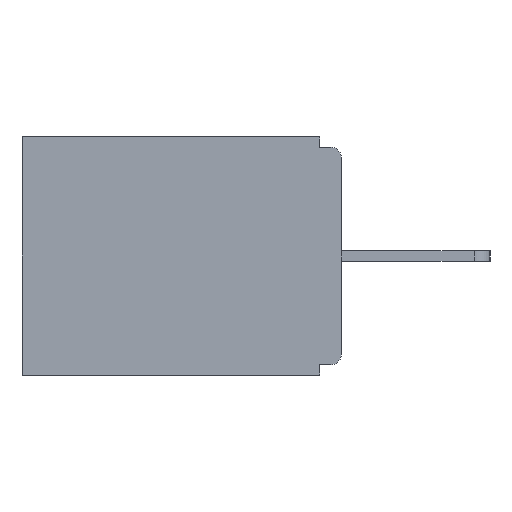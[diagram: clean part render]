
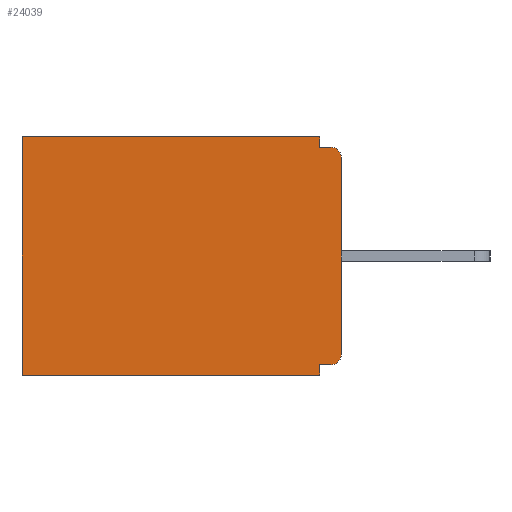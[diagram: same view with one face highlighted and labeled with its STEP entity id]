
A CAD part, left-side view. The second image highlights one B-rep face of the part: STEP entity #24039.
In plain terms, the highlighted planar face has unit normal (-1, 0, 0).
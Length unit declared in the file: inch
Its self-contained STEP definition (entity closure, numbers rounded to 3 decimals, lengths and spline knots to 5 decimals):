
#53 = LINE ( 'NONE', #6033, #4845 ) ;
#126 = VECTOR ( 'NONE', #24595, 39.37008 ) ;
#134 = EDGE_LOOP ( 'NONE', ( #587, #21879, #17811, #18312, #21061, #21093, #11610, #23595, #15843, #8886 ) ) ;
#587 = ORIENTED_EDGE ( 'NONE', *, *, #18206, .T. ) ;
#593 = CARTESIAN_POINT ( 'NONE',  ( 0.298, 0.015, -0.328 ) ) ;
#1632 = EDGE_CURVE ( 'NONE', #15498, #21610, #16433, .T. ) ;
#1956 = VECTOR ( 'NONE', #16701, 39.37008 ) ;
#2041 = VERTEX_POINT ( 'NONE', #22790 ) ;
#2462 = DIRECTION ( 'NONE',  ( 0., 0., -1. ) ) ;
#2502 = VERTEX_POINT ( 'NONE', #20215 ) ;
#3595 = EDGE_CURVE ( 'NONE', #24499, #2502, #21696, .T. ) ;
#3769 = FACE_OUTER_BOUND ( 'NONE', #134, .T. ) ;
#4038 = PLANE ( 'NONE',  #14611 ) ;
#4407 = EDGE_CURVE ( 'NONE', #12067, #2502, #9379, .T. ) ;
#4606 = CARTESIAN_POINT ( 'NONE',  ( 0.298, 0.031, 0. ) ) ;
#4625 = EDGE_CURVE ( 'NONE', #16371, #12067, #24307, .T. ) ;
#4845 = VECTOR ( 'NONE', #13504, 39.37008 ) ;
#4949 = VECTOR ( 'NONE', #23212, 39.37008 ) ;
#6033 = CARTESIAN_POINT ( 'NONE',  ( 0.298, 0.031, -0.343 ) ) ;
#6102 = DIRECTION ( 'NONE',  ( 0., 0., -1. ) ) ;
#6248 = EDGE_CURVE ( 'NONE', #18153, #21610, #20789, .T. ) ;
#6457 = CARTESIAN_POINT ( 'NONE',  ( 0.298, 0., 0. ) ) ;
#6572 = DIRECTION ( 'NONE',  ( 0., 1., 0. ) ) ;
#6909 = EDGE_CURVE ( 'NONE', #2041, #24272, #15732, .T. ) ;
#7142 = CARTESIAN_POINT ( 'NONE',  ( 0.298, 0., -0.328 ) ) ;
#7146 = CARTESIAN_POINT ( 'NONE',  ( 0.298, 0., -0.03 ) ) ;
#7517 = AXIS2_PLACEMENT_3D ( 'NONE', #8905, #22947, #10972 ) ;
#7763 = EDGE_CURVE ( 'NONE', #16371, #2041, #53, .T. ) ;
#7942 = CARTESIAN_POINT ( 'NONE',  ( 0.298, 0.015, -0.313 ) ) ;
#8074 = VECTOR ( 'NONE', #2462, 39.37008 ) ;
#8426 = VERTEX_POINT ( 'NONE', #22854 ) ;
#8474 = DIRECTION ( 'NONE',  ( 0., 0., -1. ) ) ;
#8886 = ORIENTED_EDGE ( 'NONE', *, *, #1632, .F. ) ;
#8905 = CARTESIAN_POINT ( 'NONE',  ( 0.298, 0.015, -0.03 ) ) ;
#9199 = EDGE_CURVE ( 'NONE', #8426, #24499, #18119, .T. ) ;
#9379 = LINE ( 'NONE', #12613, #8074 ) ;
#10373 = VECTOR ( 'NONE', #16014, 39.37008 ) ;
#10446 = CARTESIAN_POINT ( 'NONE',  ( 0.298, 0.031, -0.343 ) ) ;
#10972 = DIRECTION ( 'NONE',  ( 0., 0., -1. ) ) ;
#11020 = CARTESIAN_POINT ( 'NONE',  ( 0.298, 0.015, -0.015 ) ) ;
#11089 = VECTOR ( 'NONE', #8474, 39.37008 ) ;
#11223 = CARTESIAN_POINT ( 'NONE',  ( 0.298, 0., 0. ) ) ;
#11610 = ORIENTED_EDGE ( 'NONE', *, *, #9199, .F. ) ;
#12067 = VERTEX_POINT ( 'NONE', #25063 ) ;
#12613 = CARTESIAN_POINT ( 'NONE',  ( 0.298, 0.46, 0. ) ) ;
#13504 = DIRECTION ( 'NONE',  ( 0., 0., -1. ) ) ;
#14611 = AXIS2_PLACEMENT_3D ( 'NONE', #25976, #18225, #6102 ) ;
#15498 = VERTEX_POINT ( 'NONE', #7146 ) ;
#15732 = LINE ( 'NONE', #17384, #10373 ) ;
#15843 = ORIENTED_EDGE ( 'NONE', *, *, #6248, .T. ) ;
#15930 = AXIS2_PLACEMENT_3D ( 'NONE', #7942, #21995, #25230 ) ;
#16014 = DIRECTION ( 'NONE',  ( 0., -1., 0. ) ) ;
#16371 = VERTEX_POINT ( 'NONE', #4606 ) ;
#16433 = LINE ( 'NONE', #11223, #11089 ) ;
#16701 = DIRECTION ( 'NONE',  ( 0., 0., -1. ) ) ;
#17384 = CARTESIAN_POINT ( 'NONE',  ( 0.298, 0., -0.015 ) ) ;
#17642 = EDGE_CURVE ( 'NONE', #18153, #8426, #21115, .T. ) ;
#17770 = CARTESIAN_POINT ( 'NONE',  ( 0.298, 0.031, -0.343 ) ) ;
#17811 = ORIENTED_EDGE ( 'NONE', *, *, #7763, .F. ) ;
#18119 = LINE ( 'NONE', #10446, #1956 ) ;
#18153 = VERTEX_POINT ( 'NONE', #593 ) ;
#18206 = EDGE_CURVE ( 'NONE', #15498, #24272, #24113, .T. ) ;
#18225 = DIRECTION ( 'NONE',  ( 1., 0., 0. ) ) ;
#18312 = ORIENTED_EDGE ( 'NONE', *, *, #4625, .T. ) ;
#19141 = VECTOR ( 'NONE', #6572, 39.37008 ) ;
#20215 = CARTESIAN_POINT ( 'NONE',  ( 0.298, 0.46, -0.343 ) ) ;
#20695 = CARTESIAN_POINT ( 'NONE',  ( 0.298, 0., -0.313 ) ) ;
#20789 = CIRCLE ( 'NONE', #15930, 0.015 ) ;
#21061 = ORIENTED_EDGE ( 'NONE', *, *, #4407, .T. ) ;
#21093 = ORIENTED_EDGE ( 'NONE', *, *, #3595, .F. ) ;
#21115 = LINE ( 'NONE', #7142, #4949 ) ;
#21335 = CARTESIAN_POINT ( 'NONE',  ( 0.298, 0., -0.343 ) ) ;
#21610 = VERTEX_POINT ( 'NONE', #20695 ) ;
#21696 = LINE ( 'NONE', #21335, #126 ) ;
#21879 = ORIENTED_EDGE ( 'NONE', *, *, #6909, .F. ) ;
#21995 = DIRECTION ( 'NONE',  ( -1., 0., 0. ) ) ;
#22790 = CARTESIAN_POINT ( 'NONE',  ( 0.298, 0.031, -0.015 ) ) ;
#22854 = CARTESIAN_POINT ( 'NONE',  ( 0.298, 0.031, -0.328 ) ) ;
#22947 = DIRECTION ( 'NONE',  ( -1., 0., 0. ) ) ;
#23212 = DIRECTION ( 'NONE',  ( 0., 1., 0. ) ) ;
#23595 = ORIENTED_EDGE ( 'NONE', *, *, #17642, .F. ) ;
#24039 = ADVANCED_FACE ( 'NONE', ( #3769 ), #4038, .F. ) ;
#24113 = CIRCLE ( 'NONE', #7517, 0.015 ) ;
#24272 = VERTEX_POINT ( 'NONE', #11020 ) ;
#24307 = LINE ( 'NONE', #6457, #19141 ) ;
#24499 = VERTEX_POINT ( 'NONE', #17770 ) ;
#24595 = DIRECTION ( 'NONE',  ( 0., 1., 0. ) ) ;
#25063 = CARTESIAN_POINT ( 'NONE',  ( 0.298, 0.46, 0. ) ) ;
#25230 = DIRECTION ( 'NONE',  ( 0., 0., -1. ) ) ;
#25976 = CARTESIAN_POINT ( 'NONE',  ( 0.298, 0., 0. ) ) ;
